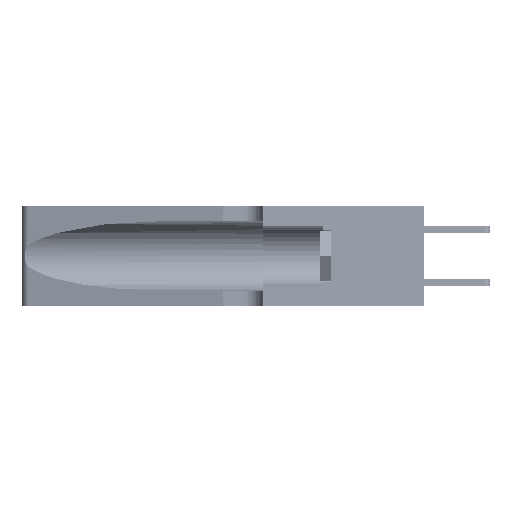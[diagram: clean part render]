
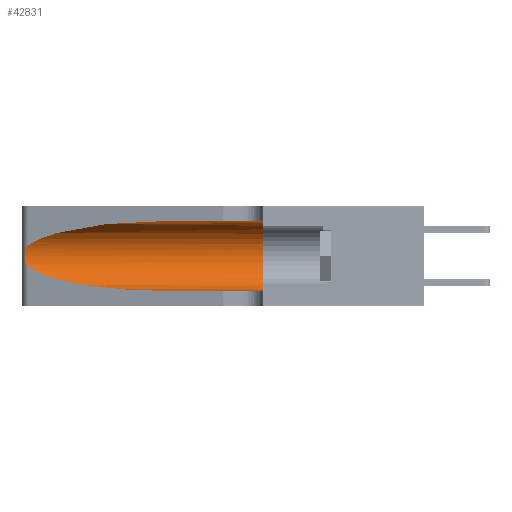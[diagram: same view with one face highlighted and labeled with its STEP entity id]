
A CAD part, left-side view. The second image highlights one B-rep face of the part: STEP entity #42831.
In plain terms, the highlighted cylindrical face has radius 3.308 mm (diameter 6.617 mm), a partial arc.
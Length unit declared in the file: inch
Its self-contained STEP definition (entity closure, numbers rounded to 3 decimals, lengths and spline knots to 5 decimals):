
#1040 = VERTEX_POINT ( 'NONE', #21135 ) ;
#2209 = CARTESIAN_POINT ( 'NONE',  ( 0.1305, 0.72297, 0.05475 ) ) ;
#3124 = VECTOR ( 'NONE', #33279, 39.37008 ) ;
#3192 = ORIENTED_EDGE ( 'NONE', *, *, #18742, .F. ) ;
#4773 = AXIS2_PLACEMENT_3D ( 'NONE', #29779, #25766, #22612 ) ;
#4792 = CARTESIAN_POINT ( 'NONE',  ( 0.25856, 1.23593, 0.16098 ) ) ;
#5813 = CARTESIAN_POINT ( 'NONE',  ( 0.2373, 1.15595, 0.28018 ) ) ;
#5886 = CYLINDRICAL_SURFACE ( 'NONE', #33670, 0.13025 ) ;
#7523 = CARTESIAN_POINT ( 'NONE',  ( 0.25487, 1.22718, 0.14631 ) ) ;
#7591 = CARTESIAN_POINT ( 'NONE',  ( 0.25555, 1.22994, 0.2215 ) ) ;
#8487 = ORIENTED_EDGE ( 'NONE', *, *, #32094, .T. ) ;
#9495 = ORIENTED_EDGE ( 'NONE', *, *, #31159, .F. ) ;
#9663 = CARTESIAN_POINT ( 'NONE',  ( 0.18966, 0.96281, 0.05475 ) ) ;
#10666 = DIRECTION ( 'NONE',  ( 0., 0., -1. ) ) ;
#12427 =( BOUNDED_CURVE ( )  B_SPLINE_CURVE ( 3, ( #38244, #41832, #9663, #16842 ),
 .UNSPECIFIED., .F., .F. ) 
 B_SPLINE_CURVE_WITH_KNOTS ( ( 4, 4 ),
 ( 3.44316, 4.71239 ),
 .UNSPECIFIED. ) 
 CURVE ( )  GEOMETRIC_REPRESENTATION_ITEM ( )  RATIONAL_B_SPLINE_CURVE ( ( 1., 0.87, 0.87, 1. ) ) 
 REPRESENTATION_ITEM ( '' )  );
#12547 = CARTESIAN_POINT ( 'NONE',  ( 0.1305, 0.72297, 0.31525 ) ) ;
#12549 = EDGE_CURVE ( 'NONE', #32311, #1040, #27564, .T. ) ;
#12817 = VERTEX_POINT ( 'NONE', #2209 ) ;
#13151 = CARTESIAN_POINT ( 'NONE',  ( 0.25487, 1.22718, 0.22369 ) ) ;
#14871 = EDGE_CURVE ( 'NONE', #12817, #29761, #22083, .T. ) ;
#15417 = CARTESIAN_POINT ( 'NONE',  ( 0.25487, 1.22718, 0.22369 ) ) ;
#16622 = CARTESIAN_POINT ( 'NONE',  ( 0.1305, 0.72297, 0.31525 ) ) ;
#16842 = CARTESIAN_POINT ( 'NONE',  ( 0.1305, 0.72297, 0.05475 ) ) ;
#16918 = CARTESIAN_POINT ( 'NONE',  ( 0.1305, 1.61858, 0.31525 ) ) ;
#17231 = CARTESIAN_POINT ( 'NONE',  ( 0.1305, 0.35, 0.05475 ) ) ;
#17546 = CARTESIAN_POINT ( 'NONE',  ( 0.1305, 1.61858, 0.185 ) ) ;
#18213 = CARTESIAN_POINT ( 'NONE',  ( 0.1305, 1.61858, 0.05475 ) ) ;
#18250 = ORIENTED_EDGE ( 'NONE', *, *, #12549, .T. ) ;
#18499 = CARTESIAN_POINT ( 'NONE',  ( 0.25639, 1.23184, 0.21858 ) ) ;
#18691 = B_SPLINE_CURVE_WITH_KNOTS ( 'NONE', 3,
 ( #15417, #7591, #18499, #40201, #36029, #39596, #43204, #43359, #25558, #4792, #36798, #30046, #26186, #19452 ),
 .UNSPECIFIED., .F., .F.,
 ( 4, 2, 2, 2, 2, 2, 4 ),
 ( 0., 0.00027, 0.00053, 0.00107, 0.0016, 0.00187, 0.00214 ),
 .UNSPECIFIED. ) ;
#18732 = CIRCLE ( 'NONE', #4773, 0.13025 ) ;
#18742 = EDGE_CURVE ( 'NONE', #32311, #28017, #45485, .T. ) ;
#19452 = CARTESIAN_POINT ( 'NONE',  ( 0.25487, 1.22718, 0.14631 ) ) ;
#20984 = DIRECTION ( 'NONE',  ( 0., -1., 0. ) ) ;
#21135 = CARTESIAN_POINT ( 'NONE',  ( 0.25487, 1.22718, 0.22369 ) ) ;
#21433 = ORIENTED_EDGE ( 'NONE', *, *, #14871, .T. ) ;
#22083 = LINE ( 'NONE', #18213, #3124 ) ;
#22237 = CARTESIAN_POINT ( 'NONE',  ( 0.1305, 0.35, 0.31525 ) ) ;
#22612 = DIRECTION ( 'NONE',  ( 0., 0., 1. ) ) ;
#24418 = VECTOR ( 'NONE', #20984, 39.37008 ) ;
#25558 = CARTESIAN_POINT ( 'NONE',  ( 0.26017, 1.23833, 0.17102 ) ) ;
#25766 = DIRECTION ( 'NONE',  ( 0., 1., 0. ) ) ;
#26186 = CARTESIAN_POINT ( 'NONE',  ( 0.25555, 1.22993, 0.14849 ) ) ;
#26623 = EDGE_CURVE ( 'NONE', #32680, #12817, #12427, .T. ) ;
#27564 =( BOUNDED_CURVE ( )  B_SPLINE_CURVE ( 3, ( #12547, #44559, #5813, #13151 ),
 .UNSPECIFIED., .F., .T. ) 
 B_SPLINE_CURVE_WITH_KNOTS ( ( 4, 4 ),
 ( 1.5708, 2.84003 ),
 .UNSPECIFIED. ) 
 CURVE ( )  GEOMETRIC_REPRESENTATION_ITEM ( )  RATIONAL_B_SPLINE_CURVE ( ( 1., 0.87, 0.87, 1. ) ) 
 REPRESENTATION_ITEM ( '' )  );
#28017 = VERTEX_POINT ( 'NONE', #22237 ) ;
#28545 = ORIENTED_EDGE ( 'NONE', *, *, #26623, .T. ) ;
#29761 = VERTEX_POINT ( 'NONE', #17231 ) ;
#29779 = CARTESIAN_POINT ( 'NONE',  ( 0.1305, 0.35, 0.185 ) ) ;
#30046 = CARTESIAN_POINT ( 'NONE',  ( 0.25639, 1.23186, 0.15144 ) ) ;
#31159 = EDGE_CURVE ( 'NONE', #28017, #29761, #18732, .T. ) ;
#32094 = EDGE_CURVE ( 'NONE', #1040, #32680, #18691, .T. ) ;
#32311 = VERTEX_POINT ( 'NONE', #16622 ) ;
#32680 = VERTEX_POINT ( 'NONE', #7523 ) ;
#33279 = DIRECTION ( 'NONE',  ( 0., -1., 0. ) ) ;
#33670 = AXIS2_PLACEMENT_3D ( 'NONE', #17546, #35548, #10666 ) ;
#35548 = DIRECTION ( 'NONE',  ( 0., -1., 0. ) ) ;
#36029 = CARTESIAN_POINT ( 'NONE',  ( 0.25854, 1.2359, 0.20912 ) ) ;
#36798 = CARTESIAN_POINT ( 'NONE',  ( 0.25789, 1.23486, 0.15765 ) ) ;
#38244 = CARTESIAN_POINT ( 'NONE',  ( 0.25487, 1.22718, 0.14631 ) ) ;
#39596 = CARTESIAN_POINT ( 'NONE',  ( 0.26018, 1.23835, 0.19895 ) ) ;
#40201 = CARTESIAN_POINT ( 'NONE',  ( 0.25787, 1.23484, 0.2124 ) ) ;
#41832 = CARTESIAN_POINT ( 'NONE',  ( 0.2373, 1.15595, 0.08982 ) ) ;
#42831 = ADVANCED_FACE ( 'NONE', ( #44851 ), #5886, .F. ) ;
#43204 = CARTESIAN_POINT ( 'NONE',  ( 0.26075, 1.23896, 0.19203 ) ) ;
#43359 = CARTESIAN_POINT ( 'NONE',  ( 0.26075, 1.23896, 0.178 ) ) ;
#44492 = EDGE_LOOP ( 'NONE', ( #18250, #8487, #28545, #21433, #9495, #3192 ) ) ;
#44559 = CARTESIAN_POINT ( 'NONE',  ( 0.18966, 0.96281, 0.31525 ) ) ;
#44851 = FACE_OUTER_BOUND ( 'NONE', #44492, .T. ) ;
#45485 = LINE ( 'NONE', #16918, #24418 ) ;
